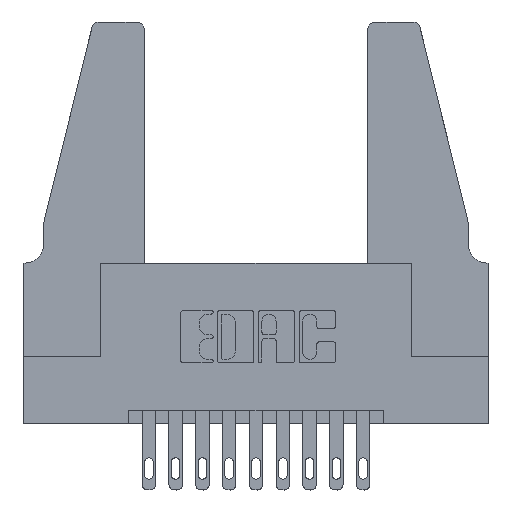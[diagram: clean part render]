
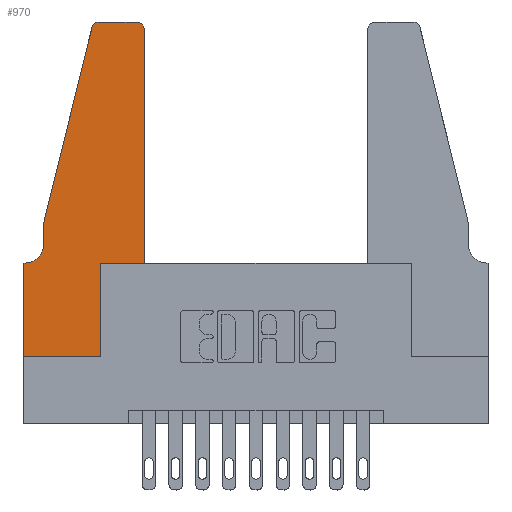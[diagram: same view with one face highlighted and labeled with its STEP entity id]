
A CAD part, top view. The second image highlights one B-rep face of the part: STEP entity #970.
In plain terms, the highlighted planar face has unit normal (0, 0, 1).
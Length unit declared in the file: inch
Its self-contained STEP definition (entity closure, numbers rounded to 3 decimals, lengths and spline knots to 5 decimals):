
#57 = DIRECTION ( 'NONE',  ( 0., 1., 0. ) ) ;
#88 = EDGE_CURVE ( 'NONE', #4899, #10336, #13226, .T. ) ;
#148 = EDGE_CURVE ( 'NONE', #5954, #1130, #11578, .T. ) ;
#185 = CARTESIAN_POINT ( 'NONE',  ( 0., 0.35, 0.37 ) ) ;
#226 = VERTEX_POINT ( 'NONE', #12482 ) ;
#318 = AXIS2_PLACEMENT_3D ( 'NONE', #1954, #10387, #8297 ) ;
#643 = DIRECTION ( 'NONE',  ( 1., 0., 0. ) ) ;
#762 = CARTESIAN_POINT ( 'NONE',  ( 0.0755, 0.5, 0.37 ) ) ;
#800 = CARTESIAN_POINT ( 'NONE',  ( 0., 0., 0.37 ) ) ;
#955 = LINE ( 'NONE', #5637, #5554 ) ;
#970 = ADVANCED_FACE ( 'NONE', ( #7471 ), #5305, .T. ) ;
#1130 = VERTEX_POINT ( 'NONE', #185 ) ;
#1271 = ORIENTED_EDGE ( 'NONE', *, *, #5784, .T. ) ;
#1358 = LINE ( 'NONE', #6370, #8112 ) ;
#1526 = LINE ( 'NONE', #800, #11719 ) ;
#1630 = CARTESIAN_POINT ( 'NONE',  ( 0., 0., 0.37 ) ) ;
#1748 = DIRECTION ( 'NONE',  ( 1., 0., 0. ) ) ;
#1859 = AXIS2_PLACEMENT_3D ( 'NONE', #2755, #4770, #1748 ) ;
#1954 = CARTESIAN_POINT ( 'NONE',  ( 0., 0.35, 0.37 ) ) ;
#2412 = LINE ( 'NONE', #2918, #10455 ) ;
#2626 = ORIENTED_EDGE ( 'NONE', *, *, #7190, .T. ) ;
#2683 = EDGE_CURVE ( 'NONE', #13077, #7905, #2412, .T. ) ;
#2739 = DIRECTION ( 'NONE',  ( 1., 0., 0. ) ) ;
#2755 = CARTESIAN_POINT ( 'NONE',  ( 0.4205, 1.22, 0.37 ) ) ;
#2791 = AXIS2_PLACEMENT_3D ( 'NONE', #7146, #13550, #12364 ) ;
#2918 = CARTESIAN_POINT ( 'NONE',  ( 0., 0., 0.37 ) ) ;
#3089 = CARTESIAN_POINT ( 'NONE',  ( 0.2865, 0., 0.37 ) ) ;
#3155 = ORIENTED_EDGE ( 'NONE', *, *, #10825, .T. ) ;
#3276 = VECTOR ( 'NONE', #11141, 39.37008 ) ;
#3444 = VERTEX_POINT ( 'NONE', #9015 ) ;
#3460 = CARTESIAN_POINT ( 'NONE',  ( 0.0755, 0.42, 0.37 ) ) ;
#3660 = DIRECTION ( 'NONE',  ( 1., 0., 0. ) ) ;
#3721 = CARTESIAN_POINT ( 'NONE',  ( 0.0755, 0.5, 0.37 ) ) ;
#3785 = VECTOR ( 'NONE', #6042, 39.37008 ) ;
#3927 = DIRECTION ( 'NONE',  ( 0., -1., 0. ) ) ;
#4245 = EDGE_CURVE ( 'NONE', #10336, #3444, #9307, .T. ) ;
#4538 = CARTESIAN_POINT ( 'NONE',  ( 0.0755, 0.35, 0.37 ) ) ;
#4770 = DIRECTION ( 'NONE',  ( 0., 0., 1. ) ) ;
#4899 = VERTEX_POINT ( 'NONE', #8469 ) ;
#4964 = DIRECTION ( 'NONE',  ( 0., -1., 0. ) ) ;
#4967 = VECTOR ( 'NONE', #4964, 39.37008 ) ;
#5189 = VECTOR ( 'NONE', #8777, 39.37008 ) ;
#5209 = CIRCLE ( 'NONE', #1859, 0.03 ) ;
#5305 = PLANE ( 'NONE',  #318 ) ;
#5457 = ORIENTED_EDGE ( 'NONE', *, *, #10044, .T. ) ;
#5530 = EDGE_CURVE ( 'NONE', #1130, #13077, #1526, .T. ) ;
#5554 = VECTOR ( 'NONE', #3660, 39.37008 ) ;
#5637 = CARTESIAN_POINT ( 'NONE',  ( 0.4505, 0.35, 0.37 ) ) ;
#5784 = EDGE_CURVE ( 'NONE', #7905, #226, #1358, .T. ) ;
#5954 = VERTEX_POINT ( 'NONE', #11645 ) ;
#6042 = DIRECTION ( 'NONE',  ( 0., 1., 0. ) ) ;
#6072 = CARTESIAN_POINT ( 'NONE',  ( 0.0755, 0.5, 0.37 ) ) ;
#6075 = LINE ( 'NONE', #3721, #3276 ) ;
#6370 = CARTESIAN_POINT ( 'NONE',  ( 0.2865, 0.35, 0.37 ) ) ;
#6424 = EDGE_CURVE ( 'NONE', #7644, #13434, #7278, .T. ) ;
#6458 = CARTESIAN_POINT ( 'NONE',  ( 0.4505, 1.22, 0.37 ) ) ;
#6764 = ORIENTED_EDGE ( 'NONE', *, *, #4245, .T. ) ;
#6863 = ORIENTED_EDGE ( 'NONE', *, *, #12361, .T. ) ;
#7146 = CARTESIAN_POINT ( 'NONE',  ( 0.0055, 0.42, 0.37 ) ) ;
#7190 = EDGE_CURVE ( 'NONE', #8140, #11785, #11498, .T. ) ;
#7278 = LINE ( 'NONE', #6072, #4967 ) ;
#7345 = AXIS2_PLACEMENT_3D ( 'NONE', #13362, #10168, #643 ) ;
#7471 = FACE_OUTER_BOUND ( 'NONE', #8600, .T. ) ;
#7644 = VERTEX_POINT ( 'NONE', #762 ) ;
#7750 = ORIENTED_EDGE ( 'NONE', *, *, #148, .T. ) ;
#7905 = VERTEX_POINT ( 'NONE', #3089 ) ;
#8111 = CARTESIAN_POINT ( 'NONE',  ( 0.4505, 0.35, 0.37 ) ) ;
#8112 = VECTOR ( 'NONE', #57, 39.37008 ) ;
#8140 = VERTEX_POINT ( 'NONE', #8624 ) ;
#8204 = ORIENTED_EDGE ( 'NONE', *, *, #88, .T. ) ;
#8297 = DIRECTION ( 'NONE',  ( 1., 0., 0. ) ) ;
#8469 = CARTESIAN_POINT ( 'NONE',  ( 0.4205, 1.25, 0.37 ) ) ;
#8600 = EDGE_LOOP ( 'NONE', ( #8204, #6764, #3155, #12921, #5457, #7750, #9272, #9253, #1271, #11227, #2626, #6863 ) ) ;
#8624 = CARTESIAN_POINT ( 'NONE',  ( 0.4505, 0.35, 0.37 ) ) ;
#8777 = DIRECTION ( 'NONE',  ( -1., 0., 0. ) ) ;
#8804 = VECTOR ( 'NONE', #9734, 39.37008 ) ;
#9015 = CARTESIAN_POINT ( 'NONE',  ( 0.25487, 1.22718, 0.37 ) ) ;
#9102 = CARTESIAN_POINT ( 'NONE',  ( 0.284, 1.25, 0.37 ) ) ;
#9253 = ORIENTED_EDGE ( 'NONE', *, *, #2683, .T. ) ;
#9272 = ORIENTED_EDGE ( 'NONE', *, *, #5530, .T. ) ;
#9307 = CIRCLE ( 'NONE', #7345, 0.03 ) ;
#9734 = DIRECTION ( 'NONE',  ( -1., 0., 0. ) ) ;
#10044 = EDGE_CURVE ( 'NONE', #13434, #5954, #10503, .T. ) ;
#10168 = DIRECTION ( 'NONE',  ( 0., 0., 1. ) ) ;
#10336 = VERTEX_POINT ( 'NONE', #9102 ) ;
#10387 = DIRECTION ( 'NONE',  ( 0., 0., 1. ) ) ;
#10455 = VECTOR ( 'NONE', #2739, 39.37008 ) ;
#10503 = CIRCLE ( 'NONE', #2791, 0.07 ) ;
#10825 = EDGE_CURVE ( 'NONE', #3444, #7644, #6075, .T. ) ;
#11141 = DIRECTION ( 'NONE',  ( -0.239, -0.971, 0. ) ) ;
#11227 = ORIENTED_EDGE ( 'NONE', *, *, #11495, .T. ) ;
#11495 = EDGE_CURVE ( 'NONE', #226, #8140, #955, .T. ) ;
#11498 = LINE ( 'NONE', #8111, #3785 ) ;
#11578 = LINE ( 'NONE', #4538, #8804 ) ;
#11645 = CARTESIAN_POINT ( 'NONE',  ( 0.0055, 0.35, 0.37 ) ) ;
#11719 = VECTOR ( 'NONE', #3927, 39.37008 ) ;
#11785 = VERTEX_POINT ( 'NONE', #6458 ) ;
#12361 = EDGE_CURVE ( 'NONE', #11785, #4899, #5209, .T. ) ;
#12364 = DIRECTION ( 'NONE',  ( -1., 0., 0. ) ) ;
#12482 = CARTESIAN_POINT ( 'NONE',  ( 0.2865, 0.35, 0.37 ) ) ;
#12734 = CARTESIAN_POINT ( 'NONE',  ( 0.2605, 1.25, 0.37 ) ) ;
#12921 = ORIENTED_EDGE ( 'NONE', *, *, #6424, .T. ) ;
#13077 = VERTEX_POINT ( 'NONE', #1630 ) ;
#13226 = LINE ( 'NONE', #12734, #5189 ) ;
#13362 = CARTESIAN_POINT ( 'NONE',  ( 0.284, 1.22, 0.37 ) ) ;
#13434 = VERTEX_POINT ( 'NONE', #3460 ) ;
#13550 = DIRECTION ( 'NONE',  ( 0., 0., -1. ) ) ;
